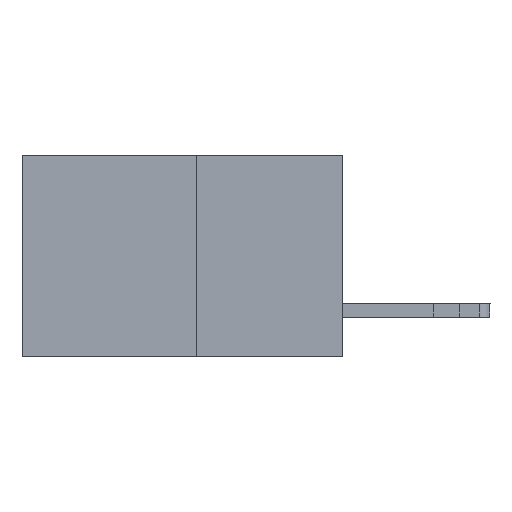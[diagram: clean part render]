
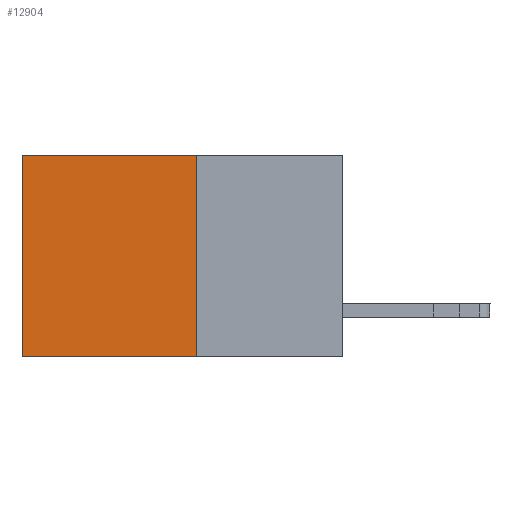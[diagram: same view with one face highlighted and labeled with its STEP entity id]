
A CAD part, left-side view. The second image highlights one B-rep face of the part: STEP entity #12904.
In plain terms, the highlighted planar face has unit normal (-1, 0, 0).
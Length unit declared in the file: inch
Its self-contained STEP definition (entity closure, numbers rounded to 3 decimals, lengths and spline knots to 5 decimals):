
#363 = DIRECTION ( 'NONE',  ( 1., 0., 0. ) ) ;
#509 = EDGE_CURVE ( 'NONE', #1766, #9343, #8563, .T. ) ;
#777 = AXIS2_PLACEMENT_3D ( 'NONE', #7628, #363, #8879 ) ;
#939 = ORIENTED_EDGE ( 'NONE', *, *, #3084, .T. ) ;
#1766 = VERTEX_POINT ( 'NONE', #14303 ) ;
#1773 = CARTESIAN_POINT ( 'NONE',  ( 0.277, 0.27, 0. ) ) ;
#2125 = VERTEX_POINT ( 'NONE', #11653 ) ;
#2234 = VERTEX_POINT ( 'NONE', #10486 ) ;
#2295 = ORIENTED_EDGE ( 'NONE', *, *, #12885, .F. ) ;
#2316 = CARTESIAN_POINT ( 'NONE',  ( 0.277, 0.27, -0.37 ) ) ;
#2718 = ORIENTED_EDGE ( 'NONE', *, *, #7192, .F. ) ;
#2731 = DIRECTION ( 'NONE',  ( 0., 0., -1. ) ) ;
#2741 = CARTESIAN_POINT ( 'NONE',  ( 0.277, 0.59, -0.37 ) ) ;
#3084 = EDGE_CURVE ( 'NONE', #9343, #2234, #3366, .T. ) ;
#3366 = LINE ( 'NONE', #2741, #9422 ) ;
#5175 = LINE ( 'NONE', #2316, #13608 ) ;
#6466 = PLANE ( 'NONE',  #777 ) ;
#7192 = EDGE_CURVE ( 'NONE', #1766, #2125, #5175, .T. ) ;
#7628 = CARTESIAN_POINT ( 'NONE',  ( 0.277, 0.27, -0.37 ) ) ;
#8168 = DIRECTION ( 'NONE',  ( 0., 1., 0. ) ) ;
#8563 = LINE ( 'NONE', #1773, #14493 ) ;
#8879 = DIRECTION ( 'NONE',  ( 0., 0., -1. ) ) ;
#9305 = VECTOR ( 'NONE', #10028, 39.37008 ) ;
#9343 = VERTEX_POINT ( 'NONE', #13921 ) ;
#9422 = VECTOR ( 'NONE', #2731, 39.37008 ) ;
#9686 = LINE ( 'NONE', #11216, #9305 ) ;
#9690 = EDGE_LOOP ( 'NONE', ( #939, #2295, #2718, #14232 ) ) ;
#10028 = DIRECTION ( 'NONE',  ( 0., 1., 0. ) ) ;
#10486 = CARTESIAN_POINT ( 'NONE',  ( 0.277, 0.59, -0.37 ) ) ;
#11216 = CARTESIAN_POINT ( 'NONE',  ( 0.277, 0.27, -0.37 ) ) ;
#11653 = CARTESIAN_POINT ( 'NONE',  ( 0.277, 0.27, -0.37 ) ) ;
#12885 = EDGE_CURVE ( 'NONE', #2125, #2234, #9686, .T. ) ;
#12904 = ADVANCED_FACE ( 'NONE', ( #15239 ), #6466, .F. ) ;
#13608 = VECTOR ( 'NONE', #14311, 39.37008 ) ;
#13921 = CARTESIAN_POINT ( 'NONE',  ( 0.277, 0.59, 0. ) ) ;
#14232 = ORIENTED_EDGE ( 'NONE', *, *, #509, .T. ) ;
#14303 = CARTESIAN_POINT ( 'NONE',  ( 0.277, 0.27, 0. ) ) ;
#14311 = DIRECTION ( 'NONE',  ( 0., 0., -1. ) ) ;
#14493 = VECTOR ( 'NONE', #8168, 39.37008 ) ;
#15239 = FACE_OUTER_BOUND ( 'NONE', #9690, .T. ) ;
